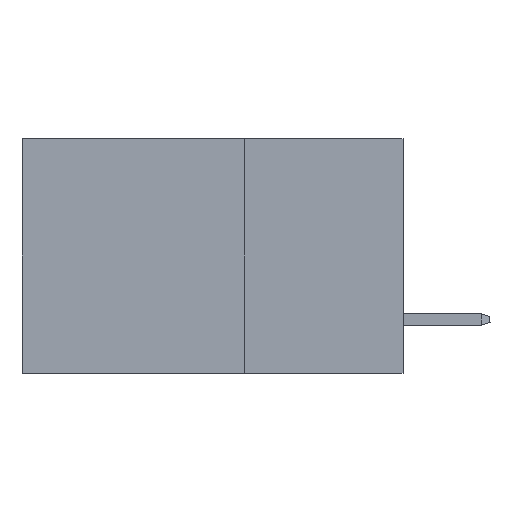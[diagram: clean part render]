
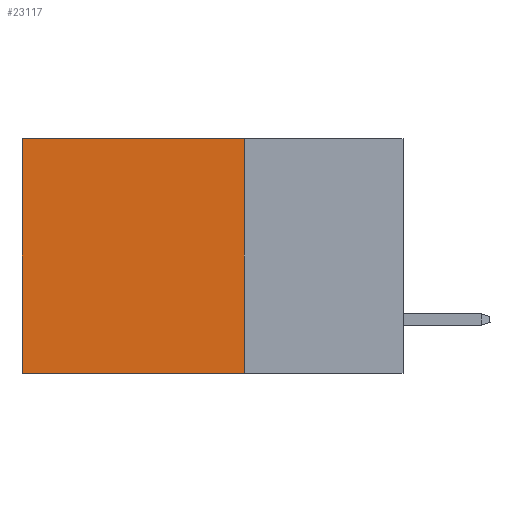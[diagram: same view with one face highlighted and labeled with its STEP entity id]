
A CAD part, left-side view. The second image highlights one B-rep face of the part: STEP entity #23117.
In plain terms, the highlighted planar face has unit normal (-1, 0, 0).
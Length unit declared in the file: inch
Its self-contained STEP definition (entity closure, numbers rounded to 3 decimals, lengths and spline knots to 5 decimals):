
#392 = ORIENTED_EDGE ( 'NONE', *, *, #29233, .T. ) ;
#2262 = VERTEX_POINT ( 'NONE', #4712 ) ;
#2978 = DIRECTION ( 'NONE',  ( 1., 0., 0. ) ) ;
#4381 = ORIENTED_EDGE ( 'NONE', *, *, #28981, .F. ) ;
#4448 = CARTESIAN_POINT ( 'NONE',  ( 0.2875, 0.6, 0. ) ) ;
#4500 = VERTEX_POINT ( 'NONE', #20026 ) ;
#4712 = CARTESIAN_POINT ( 'NONE',  ( 0.2875, 0.25, -0.37 ) ) ;
#5464 = DIRECTION ( 'NONE',  ( 0., 1., 0. ) ) ;
#5747 = VECTOR ( 'NONE', #28703, 39.37008 ) ;
#5941 = CARTESIAN_POINT ( 'NONE',  ( 0.2875, 0.25, 0. ) ) ;
#10360 = DIRECTION ( 'NONE',  ( 0., 0., -1. ) ) ;
#10453 = VERTEX_POINT ( 'NONE', #36652 ) ;
#11283 = CARTESIAN_POINT ( 'NONE',  ( 0.2875, 0.25, 0. ) ) ;
#13902 = CARTESIAN_POINT ( 'NONE',  ( 0.2875, 0.25, 0. ) ) ;
#14357 = LINE ( 'NONE', #32585, #37851 ) ;
#16720 = ORIENTED_EDGE ( 'NONE', *, *, #30911, .T. ) ;
#18895 = EDGE_CURVE ( 'NONE', #26155, #2262, #30492, .T. ) ;
#20026 = CARTESIAN_POINT ( 'NONE',  ( 0.2875, 0.6, 0. ) ) ;
#20812 = VECTOR ( 'NONE', #28108, 39.37008 ) ;
#21357 = FACE_OUTER_BOUND ( 'NONE', #37476, .T. ) ;
#23117 = ADVANCED_FACE ( 'NONE', ( #21357 ), #24318, .F. ) ;
#24318 = PLANE ( 'NONE',  #24341 ) ;
#24341 = AXIS2_PLACEMENT_3D ( 'NONE', #5941, #2978, #30464 ) ;
#26155 = VERTEX_POINT ( 'NONE', #13902 ) ;
#28108 = DIRECTION ( 'NONE',  ( 0., 0., -1. ) ) ;
#28703 = DIRECTION ( 'NONE',  ( 0., 1., 0. ) ) ;
#28981 = EDGE_CURVE ( 'NONE', #2262, #10453, #14357, .T. ) ;
#29233 = EDGE_CURVE ( 'NONE', #4500, #10453, #35094, .T. ) ;
#30464 = DIRECTION ( 'NONE',  ( 0., 0., -1. ) ) ;
#30492 = LINE ( 'NONE', #31085, #20812 ) ;
#30911 = EDGE_CURVE ( 'NONE', #26155, #4500, #37616, .T. ) ;
#31085 = CARTESIAN_POINT ( 'NONE',  ( 0.2875, 0.25, 0. ) ) ;
#32585 = CARTESIAN_POINT ( 'NONE',  ( 0.2875, 0.25, -0.37 ) ) ;
#35094 = LINE ( 'NONE', #4448, #37242 ) ;
#36652 = CARTESIAN_POINT ( 'NONE',  ( 0.2875, 0.6, -0.37 ) ) ;
#37242 = VECTOR ( 'NONE', #10360, 39.37008 ) ;
#37476 = EDGE_LOOP ( 'NONE', ( #392, #4381, #37592, #16720 ) ) ;
#37592 = ORIENTED_EDGE ( 'NONE', *, *, #18895, .F. ) ;
#37616 = LINE ( 'NONE', #11283, #5747 ) ;
#37851 = VECTOR ( 'NONE', #5464, 39.37008 ) ;
